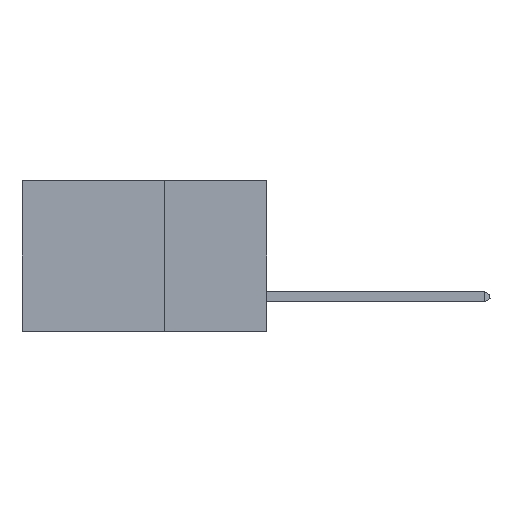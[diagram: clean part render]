
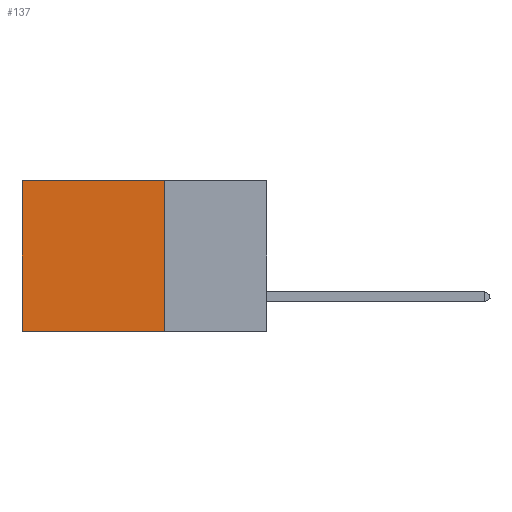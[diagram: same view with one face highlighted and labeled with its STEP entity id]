
A CAD part, left-side view. The second image highlights one B-rep face of the part: STEP entity #137.
In plain terms, the highlighted planar face has unit normal (-1, 0, 0).
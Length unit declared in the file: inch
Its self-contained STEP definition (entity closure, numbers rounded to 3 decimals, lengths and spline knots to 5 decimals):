
#137 = ADVANCED_FACE ( 'NONE', ( #23692 ), #23545, .F. ) ;
#1026 = ORIENTED_EDGE ( 'NONE', *, *, #16719, .T. ) ;
#2180 = AXIS2_PLACEMENT_3D ( 'NONE', #17248, #17593, #21608 ) ;
#3351 = DIRECTION ( 'NONE',  ( 0., 1., 0. ) ) ;
#4765 = CARTESIAN_POINT ( 'NONE',  ( 0.2875, 0.25, 0. ) ) ;
#6108 = LINE ( 'NONE', #4765, #21501 ) ;
#6329 = CARTESIAN_POINT ( 'NONE',  ( 0.2875, 0.6, 0. ) ) ;
#7988 = EDGE_LOOP ( 'NONE', ( #12169, #8233, #9722, #1026 ) ) ;
#8093 = EDGE_CURVE ( 'NONE', #10377, #18694, #16749, .T. ) ;
#8233 = ORIENTED_EDGE ( 'NONE', *, *, #8093, .F. ) ;
#9185 = CARTESIAN_POINT ( 'NONE',  ( 0.2875, 0.6, -0.37 ) ) ;
#9722 = ORIENTED_EDGE ( 'NONE', *, *, #12925, .F. ) ;
#10377 = VERTEX_POINT ( 'NONE', #24255 ) ;
#10978 = DIRECTION ( 'NONE',  ( 0., 1., 0. ) ) ;
#11411 = VERTEX_POINT ( 'NONE', #23462 ) ;
#12169 = ORIENTED_EDGE ( 'NONE', *, *, #24292, .T. ) ;
#12561 = LINE ( 'NONE', #24373, #16024 ) ;
#12925 = EDGE_CURVE ( 'NONE', #25380, #10377, #6108, .T. ) ;
#13365 = LINE ( 'NONE', #6329, #14011 ) ;
#14011 = VECTOR ( 'NONE', #22388, 39.37008 ) ;
#15585 = DIRECTION ( 'NONE',  ( 0., 0., -1. ) ) ;
#16024 = VECTOR ( 'NONE', #10978, 39.37008 ) ;
#16719 = EDGE_CURVE ( 'NONE', #25380, #11411, #12561, .T. ) ;
#16749 = LINE ( 'NONE', #21282, #17688 ) ;
#17248 = CARTESIAN_POINT ( 'NONE',  ( 0.2875, 0.25, 0. ) ) ;
#17593 = DIRECTION ( 'NONE',  ( 1., 0., 0. ) ) ;
#17688 = VECTOR ( 'NONE', #3351, 39.37008 ) ;
#18694 = VERTEX_POINT ( 'NONE', #9185 ) ;
#19759 = CARTESIAN_POINT ( 'NONE',  ( 0.2875, 0.25, 0. ) ) ;
#21282 = CARTESIAN_POINT ( 'NONE',  ( 0.2875, 0.25, -0.37 ) ) ;
#21501 = VECTOR ( 'NONE', #15585, 39.37008 ) ;
#21608 = DIRECTION ( 'NONE',  ( 0., 0., -1. ) ) ;
#22388 = DIRECTION ( 'NONE',  ( 0., 0., -1. ) ) ;
#23462 = CARTESIAN_POINT ( 'NONE',  ( 0.2875, 0.6, 0. ) ) ;
#23545 = PLANE ( 'NONE',  #2180 ) ;
#23692 = FACE_OUTER_BOUND ( 'NONE', #7988, .T. ) ;
#24255 = CARTESIAN_POINT ( 'NONE',  ( 0.2875, 0.25, -0.37 ) ) ;
#24292 = EDGE_CURVE ( 'NONE', #11411, #18694, #13365, .T. ) ;
#24373 = CARTESIAN_POINT ( 'NONE',  ( 0.2875, 0.25, 0. ) ) ;
#25380 = VERTEX_POINT ( 'NONE', #19759 ) ;
